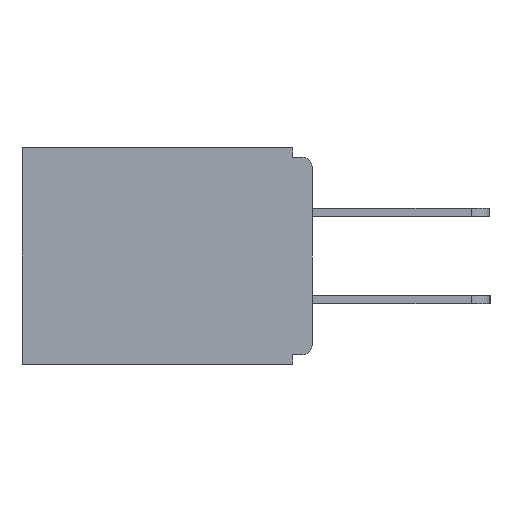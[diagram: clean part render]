
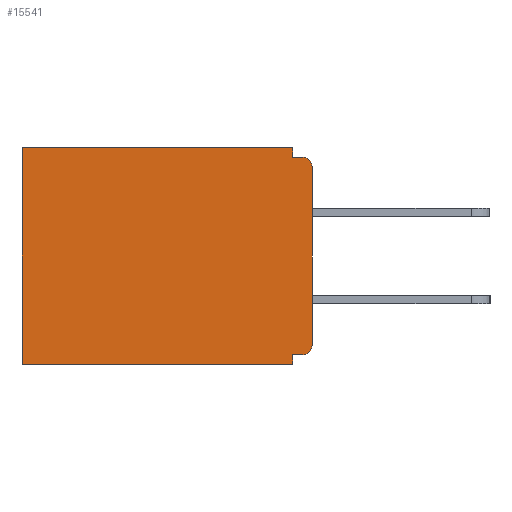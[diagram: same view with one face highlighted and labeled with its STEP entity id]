
A CAD part, left-side view. The second image highlights one B-rep face of the part: STEP entity #15541.
In plain terms, the highlighted planar face has unit normal (-1, 0, 0).
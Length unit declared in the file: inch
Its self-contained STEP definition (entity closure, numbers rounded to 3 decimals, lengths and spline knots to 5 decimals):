
#740 = EDGE_CURVE ( 'NONE', #10862, #8166, #2880, .T. ) ;
#762 = CARTESIAN_POINT ( 'NONE',  ( 0.298, 0.015, -0.03 ) ) ;
#1002 = EDGE_CURVE ( 'NONE', #16824, #11145, #19695, .T. ) ;
#1461 = VECTOR ( 'NONE', #13458, 39.37008 ) ;
#1490 = CARTESIAN_POINT ( 'NONE',  ( 0.298, 0.031, -0.343 ) ) ;
#1573 = AXIS2_PLACEMENT_3D ( 'NONE', #16405, #10387, #12016 ) ;
#1600 = LINE ( 'NONE', #6156, #4041 ) ;
#2072 = DIRECTION ( 'NONE',  ( 0., 0., -1. ) ) ;
#2135 = CARTESIAN_POINT ( 'NONE',  ( 0.298, 0.015, -0.328 ) ) ;
#2857 = VECTOR ( 'NONE', #17807, 39.37008 ) ;
#2880 = LINE ( 'NONE', #10059, #9730 ) ;
#3284 = EDGE_CURVE ( 'NONE', #16824, #8166, #13933, .T. ) ;
#3393 = DIRECTION ( 'NONE',  ( 0., 0., -1. ) ) ;
#3756 = EDGE_CURVE ( 'NONE', #10862, #11449, #13913, .T. ) ;
#3850 = VERTEX_POINT ( 'NONE', #5677 ) ;
#3974 = PLANE ( 'NONE',  #1573 ) ;
#4041 = VECTOR ( 'NONE', #17059, 39.37008 ) ;
#4840 = EDGE_CURVE ( 'NONE', #15673, #3850, #19542, .T. ) ;
#5405 = EDGE_LOOP ( 'NONE', ( #11861, #11866, #19282, #6203, #11964, #9039, #17380, #16672, #10188, #9365 ) ) ;
#5538 = DIRECTION ( 'NONE',  ( 0., -1., 0. ) ) ;
#5677 = CARTESIAN_POINT ( 'NONE',  ( 0.298, 0.031, -0.015 ) ) ;
#6076 = AXIS2_PLACEMENT_3D ( 'NONE', #14011, #9286, #7549 ) ;
#6156 = CARTESIAN_POINT ( 'NONE',  ( 0.298, 0.031, -0.343 ) ) ;
#6203 = ORIENTED_EDGE ( 'NONE', *, *, #7672, .T. ) ;
#6661 = CARTESIAN_POINT ( 'NONE',  ( 0.298, 0., -0.313 ) ) ;
#6678 = VECTOR ( 'NONE', #18599, 39.37008 ) ;
#6775 = CARTESIAN_POINT ( 'NONE',  ( 0.298, 0.015, -0.015 ) ) ;
#7331 = CARTESIAN_POINT ( 'NONE',  ( 0.298, 0.031, -0.343 ) ) ;
#7409 = LINE ( 'NONE', #19728, #6678 ) ;
#7549 = DIRECTION ( 'NONE',  ( 0., 0., -1. ) ) ;
#7574 = CARTESIAN_POINT ( 'NONE',  ( 0.298, 0.031, 0. ) ) ;
#7672 = EDGE_CURVE ( 'NONE', #15673, #19117, #11725, .T. ) ;
#8166 = VERTEX_POINT ( 'NONE', #6661 ) ;
#8618 = LINE ( 'NONE', #11685, #11768 ) ;
#9039 = ORIENTED_EDGE ( 'NONE', *, *, #11294, .F. ) ;
#9286 = DIRECTION ( 'NONE',  ( -1., 0., 0. ) ) ;
#9365 = ORIENTED_EDGE ( 'NONE', *, *, #740, .F. ) ;
#9730 = VECTOR ( 'NONE', #14559, 39.37008 ) ;
#9847 = VERTEX_POINT ( 'NONE', #1490 ) ;
#9999 = DIRECTION ( 'NONE',  ( -1., 0., 0. ) ) ;
#10059 = CARTESIAN_POINT ( 'NONE',  ( 0.298, 0., 0. ) ) ;
#10188 = ORIENTED_EDGE ( 'NONE', *, *, #3284, .T. ) ;
#10387 = DIRECTION ( 'NONE',  ( 1., 0., 0. ) ) ;
#10500 = VERTEX_POINT ( 'NONE', #11692 ) ;
#10862 = VERTEX_POINT ( 'NONE', #14927 ) ;
#10920 = EDGE_CURVE ( 'NONE', #11145, #9847, #1600, .T. ) ;
#11145 = VERTEX_POINT ( 'NONE', #17235 ) ;
#11294 = EDGE_CURVE ( 'NONE', #9847, #10500, #7409, .T. ) ;
#11449 = VERTEX_POINT ( 'NONE', #6775 ) ;
#11483 = AXIS2_PLACEMENT_3D ( 'NONE', #762, #9999, #2072 ) ;
#11685 = CARTESIAN_POINT ( 'NONE',  ( 0.298, 0., -0.015 ) ) ;
#11692 = CARTESIAN_POINT ( 'NONE',  ( 0.298, 0.46, -0.343 ) ) ;
#11725 = LINE ( 'NONE', #12059, #19554 ) ;
#11756 = CARTESIAN_POINT ( 'NONE',  ( 0.298, 0., -0.328 ) ) ;
#11768 = VECTOR ( 'NONE', #5538, 39.37008 ) ;
#11861 = ORIENTED_EDGE ( 'NONE', *, *, #3756, .T. ) ;
#11866 = ORIENTED_EDGE ( 'NONE', *, *, #12395, .F. ) ;
#11964 = ORIENTED_EDGE ( 'NONE', *, *, #15091, .T. ) ;
#12016 = DIRECTION ( 'NONE',  ( 0., 0., -1. ) ) ;
#12059 = CARTESIAN_POINT ( 'NONE',  ( 0.298, 0., 0. ) ) ;
#12072 = FACE_OUTER_BOUND ( 'NONE', #5405, .T. ) ;
#12337 = LINE ( 'NONE', #12860, #15938 ) ;
#12395 = EDGE_CURVE ( 'NONE', #3850, #11449, #8618, .T. ) ;
#12860 = CARTESIAN_POINT ( 'NONE',  ( 0.298, 0.46, 0. ) ) ;
#13458 = DIRECTION ( 'NONE',  ( 0., 0., -1. ) ) ;
#13913 = CIRCLE ( 'NONE', #11483, 0.015 ) ;
#13933 = CIRCLE ( 'NONE', #6076, 0.015 ) ;
#14011 = CARTESIAN_POINT ( 'NONE',  ( 0.298, 0.015, -0.313 ) ) ;
#14559 = DIRECTION ( 'NONE',  ( 0., 0., -1. ) ) ;
#14927 = CARTESIAN_POINT ( 'NONE',  ( 0.298, 0., -0.03 ) ) ;
#15091 = EDGE_CURVE ( 'NONE', #19117, #10500, #12337, .T. ) ;
#15375 = CARTESIAN_POINT ( 'NONE',  ( 0.298, 0.46, 0. ) ) ;
#15541 = ADVANCED_FACE ( 'NONE', ( #12072 ), #3974, .F. ) ;
#15673 = VERTEX_POINT ( 'NONE', #7574 ) ;
#15938 = VECTOR ( 'NONE', #3393, 39.37008 ) ;
#16405 = CARTESIAN_POINT ( 'NONE',  ( 0.298, 0., 0. ) ) ;
#16648 = DIRECTION ( 'NONE',  ( 0., 1., 0. ) ) ;
#16672 = ORIENTED_EDGE ( 'NONE', *, *, #1002, .F. ) ;
#16824 = VERTEX_POINT ( 'NONE', #2135 ) ;
#17059 = DIRECTION ( 'NONE',  ( 0., 0., -1. ) ) ;
#17235 = CARTESIAN_POINT ( 'NONE',  ( 0.298, 0.031, -0.328 ) ) ;
#17380 = ORIENTED_EDGE ( 'NONE', *, *, #10920, .F. ) ;
#17807 = DIRECTION ( 'NONE',  ( 0., 1., 0. ) ) ;
#18599 = DIRECTION ( 'NONE',  ( 0., 1., 0. ) ) ;
#19117 = VERTEX_POINT ( 'NONE', #15375 ) ;
#19282 = ORIENTED_EDGE ( 'NONE', *, *, #4840, .F. ) ;
#19542 = LINE ( 'NONE', #7331, #1461 ) ;
#19554 = VECTOR ( 'NONE', #16648, 39.37008 ) ;
#19695 = LINE ( 'NONE', #11756, #2857 ) ;
#19728 = CARTESIAN_POINT ( 'NONE',  ( 0.298, 0., -0.343 ) ) ;
